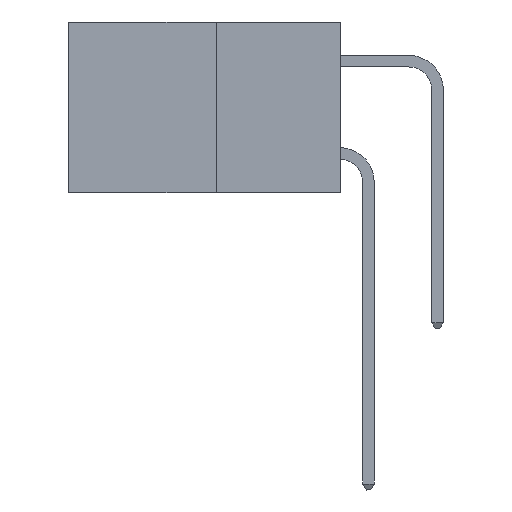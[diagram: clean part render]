
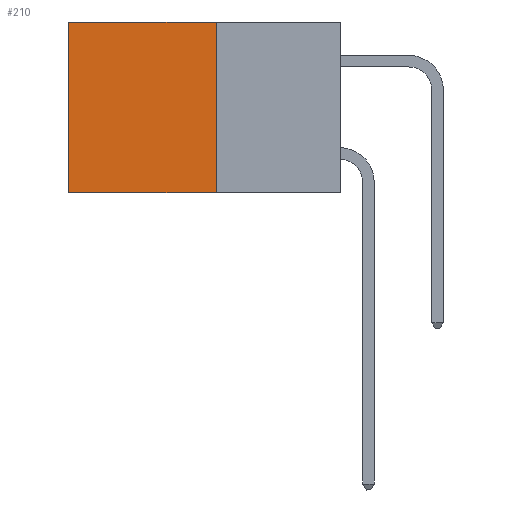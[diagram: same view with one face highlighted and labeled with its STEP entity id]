
A CAD part, left-side view. The second image highlights one B-rep face of the part: STEP entity #210.
In plain terms, the highlighted planar face has unit normal (-1, 0, 0).
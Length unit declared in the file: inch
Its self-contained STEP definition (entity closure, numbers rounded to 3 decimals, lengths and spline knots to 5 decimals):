
#186 = LINE ( 'NONE', #6429, #10459 ) ;
#210 = ADVANCED_FACE ( 'NONE', ( #7565 ), #3686, .F. ) ;
#347 = ORIENTED_EDGE ( 'NONE', *, *, #2386, .F. ) ;
#555 = VERTEX_POINT ( 'NONE', #5200 ) ;
#558 = ORIENTED_EDGE ( 'NONE', *, *, #9757, .T. ) ;
#2189 = VERTEX_POINT ( 'NONE', #7395 ) ;
#2222 = EDGE_CURVE ( 'NONE', #555, #11614, #186, .T. ) ;
#2386 = EDGE_CURVE ( 'NONE', #2189, #555, #2848, .T. ) ;
#2627 = DIRECTION ( 'NONE',  ( 0., 0., -1. ) ) ;
#2789 = CARTESIAN_POINT ( 'NONE',  ( 0.277, 0.27, -0.37 ) ) ;
#2829 = AXIS2_PLACEMENT_3D ( 'NONE', #8903, #6337, #4589 ) ;
#2848 = LINE ( 'NONE', #2789, #10307 ) ;
#3446 = EDGE_CURVE ( 'NONE', #6976, #11614, #8480, .T. ) ;
#3686 = PLANE ( 'NONE',  #2829 ) ;
#4018 = CARTESIAN_POINT ( 'NONE',  ( 0.277, 0.59, -0.37 ) ) ;
#4128 = DIRECTION ( 'NONE',  ( 0., 0., -1. ) ) ;
#4589 = DIRECTION ( 'NONE',  ( 0., 0., -1. ) ) ;
#4649 = ORIENTED_EDGE ( 'NONE', *, *, #3446, .T. ) ;
#5200 = CARTESIAN_POINT ( 'NONE',  ( 0.277, 0.27, -0.37 ) ) ;
#5334 = VECTOR ( 'NONE', #7001, 39.37008 ) ;
#5993 = DIRECTION ( 'NONE',  ( 0., 1., 0. ) ) ;
#6337 = DIRECTION ( 'NONE',  ( 1., 0., 0. ) ) ;
#6429 = CARTESIAN_POINT ( 'NONE',  ( 0.277, 0.27, -0.37 ) ) ;
#6976 = VERTEX_POINT ( 'NONE', #9759 ) ;
#7001 = DIRECTION ( 'NONE',  ( 0., 1., 0. ) ) ;
#7395 = CARTESIAN_POINT ( 'NONE',  ( 0.277, 0.27, 0. ) ) ;
#7565 = FACE_OUTER_BOUND ( 'NONE', #9874, .T. ) ;
#7977 = CARTESIAN_POINT ( 'NONE',  ( 0.277, 0.27, 0. ) ) ;
#8480 = LINE ( 'NONE', #4018, #10736 ) ;
#8797 = CARTESIAN_POINT ( 'NONE',  ( 0.277, 0.59, -0.37 ) ) ;
#8903 = CARTESIAN_POINT ( 'NONE',  ( 0.277, 0.27, -0.37 ) ) ;
#9757 = EDGE_CURVE ( 'NONE', #2189, #6976, #10498, .T. ) ;
#9759 = CARTESIAN_POINT ( 'NONE',  ( 0.277, 0.59, 0. ) ) ;
#9874 = EDGE_LOOP ( 'NONE', ( #4649, #11885, #347, #558 ) ) ;
#10307 = VECTOR ( 'NONE', #2627, 39.37008 ) ;
#10459 = VECTOR ( 'NONE', #5993, 39.37008 ) ;
#10498 = LINE ( 'NONE', #7977, #5334 ) ;
#10736 = VECTOR ( 'NONE', #4128, 39.37008 ) ;
#11614 = VERTEX_POINT ( 'NONE', #8797 ) ;
#11885 = ORIENTED_EDGE ( 'NONE', *, *, #2222, .F. ) ;
